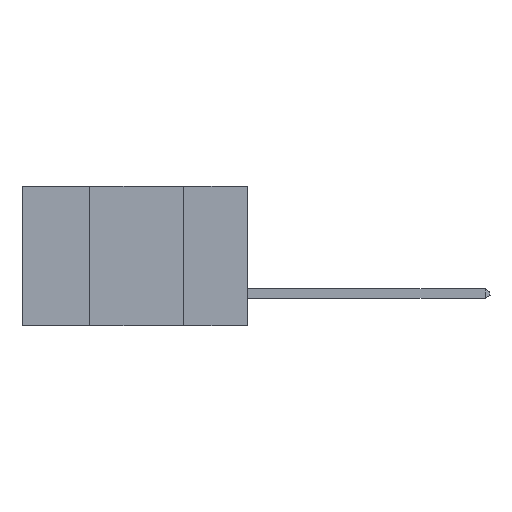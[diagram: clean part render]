
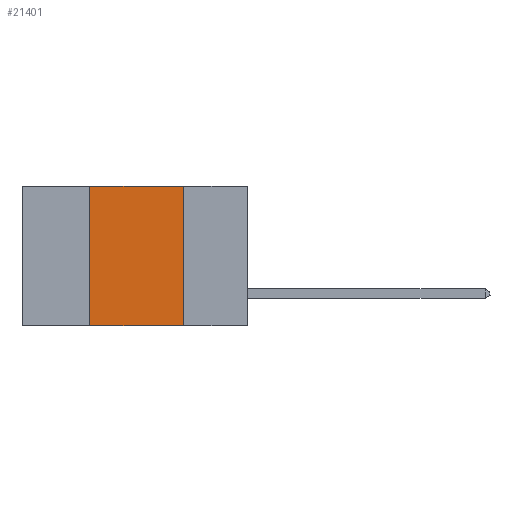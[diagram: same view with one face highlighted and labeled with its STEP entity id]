
A CAD part, left-side view. The second image highlights one B-rep face of the part: STEP entity #21401.
In plain terms, the highlighted planar face has unit normal (-1, 0, 0).
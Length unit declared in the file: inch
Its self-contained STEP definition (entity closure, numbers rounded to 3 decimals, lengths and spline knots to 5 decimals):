
#251 = CARTESIAN_POINT ( 'NONE',  ( 0., 0.42, -0.37 ) ) ;
#453 = VERTEX_POINT ( 'NONE', #3917 ) ;
#1135 = ORIENTED_EDGE ( 'NONE', *, *, #24017, .F. ) ;
#1429 = EDGE_CURVE ( 'NONE', #14586, #19849, #24083, .T. ) ;
#1473 = CARTESIAN_POINT ( 'NONE',  ( 0., 0.17, 0. ) ) ;
#1753 = CARTESIAN_POINT ( 'NONE',  ( 0., 0.42, 0. ) ) ;
#2824 = PLANE ( 'NONE',  #20486 ) ;
#3475 = EDGE_CURVE ( 'NONE', #14586, #8060, #13928, .T. ) ;
#3917 = CARTESIAN_POINT ( 'NONE',  ( 0., 0.17, 0. ) ) ;
#5346 = ORIENTED_EDGE ( 'NONE', *, *, #1429, .T. ) ;
#5947 = FACE_OUTER_BOUND ( 'NONE', #14021, .T. ) ;
#6382 = ORIENTED_EDGE ( 'NONE', *, *, #6764, .F. ) ;
#6764 = EDGE_CURVE ( 'NONE', #8060, #453, #16055, .T. ) ;
#6961 = VECTOR ( 'NONE', #16461, 39.37008 ) ;
#7257 = CARTESIAN_POINT ( 'NONE',  ( 0., 0.6, -0.37 ) ) ;
#7506 = DIRECTION ( 'NONE',  ( 0., -1., 0. ) ) ;
#7610 = VECTOR ( 'NONE', #22829, 39.37008 ) ;
#8060 = VERTEX_POINT ( 'NONE', #1753 ) ;
#8409 = ORIENTED_EDGE ( 'NONE', *, *, #3475, .F. ) ;
#9245 = CARTESIAN_POINT ( 'NONE',  ( 0., 0.6, 0. ) ) ;
#11011 = LINE ( 'NONE', #1473, #14634 ) ;
#13444 = DIRECTION ( 'NONE',  ( 0., 0., -1. ) ) ;
#13450 = VECTOR ( 'NONE', #7506, 39.37008 ) ;
#13928 = LINE ( 'NONE', #14514, #6961 ) ;
#14021 = EDGE_LOOP ( 'NONE', ( #1135, #6382, #8409, #5346 ) ) ;
#14514 = CARTESIAN_POINT ( 'NONE',  ( 0., 0.42, 0. ) ) ;
#14586 = VERTEX_POINT ( 'NONE', #251 ) ;
#14634 = VECTOR ( 'NONE', #13444, 39.37008 ) ;
#16055 = LINE ( 'NONE', #9245, #7610 ) ;
#16461 = DIRECTION ( 'NONE',  ( 0., 0., 1. ) ) ;
#18268 = CARTESIAN_POINT ( 'NONE',  ( 0., 0.6, 0. ) ) ;
#18308 = CARTESIAN_POINT ( 'NONE',  ( 0., 0.17, -0.37 ) ) ;
#18336 = DIRECTION ( 'NONE',  ( 1., 0., 0. ) ) ;
#19849 = VERTEX_POINT ( 'NONE', #18308 ) ;
#20486 = AXIS2_PLACEMENT_3D ( 'NONE', #18268, #18336, #22391 ) ;
#21401 = ADVANCED_FACE ( 'NONE', ( #5947 ), #2824, .F. ) ;
#22391 = DIRECTION ( 'NONE',  ( 0., 0., -1. ) ) ;
#22829 = DIRECTION ( 'NONE',  ( 0., -1., 0. ) ) ;
#24017 = EDGE_CURVE ( 'NONE', #453, #19849, #11011, .T. ) ;
#24083 = LINE ( 'NONE', #7257, #13450 ) ;
